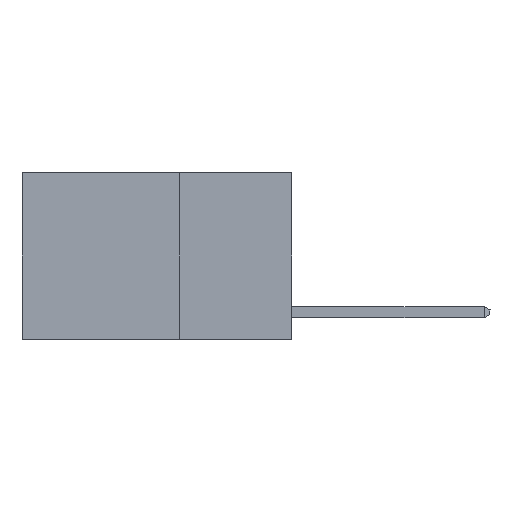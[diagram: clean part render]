
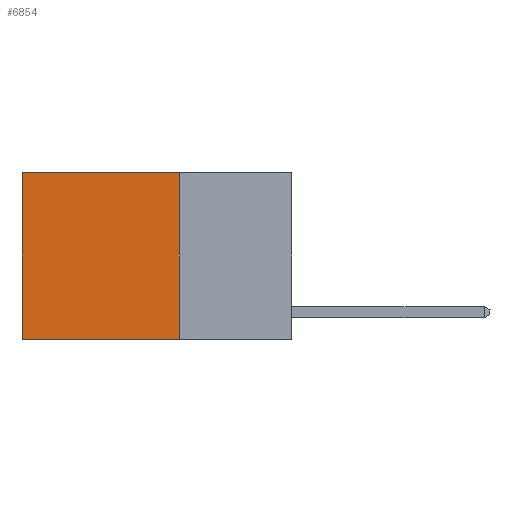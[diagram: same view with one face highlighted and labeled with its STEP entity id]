
A CAD part, left-side view. The second image highlights one B-rep face of the part: STEP entity #6854.
In plain terms, the highlighted planar face has unit normal (-1, 0, 0).
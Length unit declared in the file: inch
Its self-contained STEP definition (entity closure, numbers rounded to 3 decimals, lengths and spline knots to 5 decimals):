
#267 = CARTESIAN_POINT ( 'NONE',  ( 0.2625, 0.6, 0. ) ) ;
#822 = CARTESIAN_POINT ( 'NONE',  ( 0.2625, 0.25, 0. ) ) ;
#1218 = ORIENTED_EDGE ( 'NONE', *, *, #1894, .F. ) ;
#1610 = CARTESIAN_POINT ( 'NONE',  ( 0.2625, 0.25, 0. ) ) ;
#1891 = AXIS2_PLACEMENT_3D ( 'NONE', #1610, #5338, #7404 ) ;
#1894 = EDGE_CURVE ( 'NONE', #5682, #9494, #7645, .T. ) ;
#2270 = ORIENTED_EDGE ( 'NONE', *, *, #4899, .T. ) ;
#2426 = VECTOR ( 'NONE', #9835, 39.37008 ) ;
#2728 = VERTEX_POINT ( 'NONE', #3172 ) ;
#2785 = VERTEX_POINT ( 'NONE', #10855 ) ;
#2922 = LINE ( 'NONE', #5703, #7972 ) ;
#3066 = ORIENTED_EDGE ( 'NONE', *, *, #5080, .T. ) ;
#3172 = CARTESIAN_POINT ( 'NONE',  ( 0.2625, 0.6, -0.37 ) ) ;
#3711 = EDGE_CURVE ( 'NONE', #9494, #2728, #11644, .T. ) ;
#4066 = FACE_OUTER_BOUND ( 'NONE', #7971, .T. ) ;
#4899 = EDGE_CURVE ( 'NONE', #2785, #2728, #8613, .T. ) ;
#5080 = EDGE_CURVE ( 'NONE', #5682, #2785, #2922, .T. ) ;
#5338 = DIRECTION ( 'NONE',  ( 1., 0., 0. ) ) ;
#5482 = DIRECTION ( 'NONE',  ( 0., 0., -1. ) ) ;
#5682 = VERTEX_POINT ( 'NONE', #822 ) ;
#5703 = CARTESIAN_POINT ( 'NONE',  ( 0.2625, 0.25, 0. ) ) ;
#6119 = CARTESIAN_POINT ( 'NONE',  ( 0.2625, 0.25, 0. ) ) ;
#6854 = ADVANCED_FACE ( 'NONE', ( #4066 ), #12037, .F. ) ;
#7404 = DIRECTION ( 'NONE',  ( 0., 0., -1. ) ) ;
#7645 = LINE ( 'NONE', #6119, #2426 ) ;
#7971 = EDGE_LOOP ( 'NONE', ( #2270, #8203, #1218, #3066 ) ) ;
#7972 = VECTOR ( 'NONE', #10549, 39.37008 ) ;
#8203 = ORIENTED_EDGE ( 'NONE', *, *, #3711, .F. ) ;
#8367 = VECTOR ( 'NONE', #12108, 39.37008 ) ;
#8613 = LINE ( 'NONE', #267, #9631 ) ;
#9337 = CARTESIAN_POINT ( 'NONE',  ( 0.2625, 0.25, -0.37 ) ) ;
#9494 = VERTEX_POINT ( 'NONE', #9609 ) ;
#9609 = CARTESIAN_POINT ( 'NONE',  ( 0.2625, 0.25, -0.37 ) ) ;
#9631 = VECTOR ( 'NONE', #5482, 39.37008 ) ;
#9835 = DIRECTION ( 'NONE',  ( 0., 0., -1. ) ) ;
#10549 = DIRECTION ( 'NONE',  ( 0., 1., 0. ) ) ;
#10855 = CARTESIAN_POINT ( 'NONE',  ( 0.2625, 0.6, 0. ) ) ;
#11644 = LINE ( 'NONE', #9337, #8367 ) ;
#12037 = PLANE ( 'NONE',  #1891 ) ;
#12108 = DIRECTION ( 'NONE',  ( 0., 1., 0. ) ) ;
